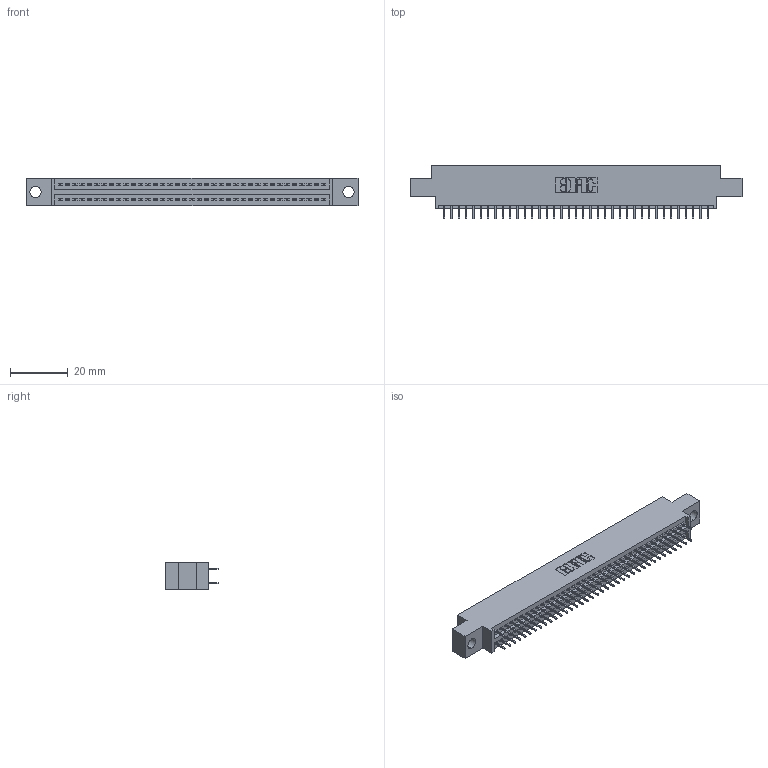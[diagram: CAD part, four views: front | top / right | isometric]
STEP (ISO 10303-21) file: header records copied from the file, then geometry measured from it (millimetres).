
FILE_DESCRIPTION (( 'STEP AP203' ), '1' );
FILE_NAME ('395-074-525-804.STEP', '2020-09-25T08:41:44', ( '' ), ( '' ), 'SwSTEP 2.0', 'SolidWorks 2020', '' );
FILE_SCHEMA (( 'CONFIG_CONTROL_DESIGN' ));
Length unit declared in the file: inch
Products named in the file (3): 345-292-001_345-293-125; 345 Part_0.170 Offset - 0.156 Dia-TH; 395-074-525-804
Assembly tree (75 placements, depth 2):
  395-074-525-804
    345 Part_0.170 Offset - 0.156 Dia-TH
    345-292-001_345-293-125  x74
Bounding box: 115.19 x 18.72 x 9.4 mm (x, y, z)
Volume: 10820.1 mm3; surface area: 15488.7 mm2
Topology: 75 solids, 75 shells, 4126 faces, 11675 edges, 7486 vertices
Faces by surface type: plane 2970, cylinder 1156
Entity records: 29913 total; most frequent: CARTESIAN_POINT 5020, ORIENTED_EDGE 4954, DIRECTION 4433, EDGE_CURVE 2477, VECTOR 2201, LINE 2201, VERTEX_POINT 1646, AXIS2_PLACEMENT_3D 1116
